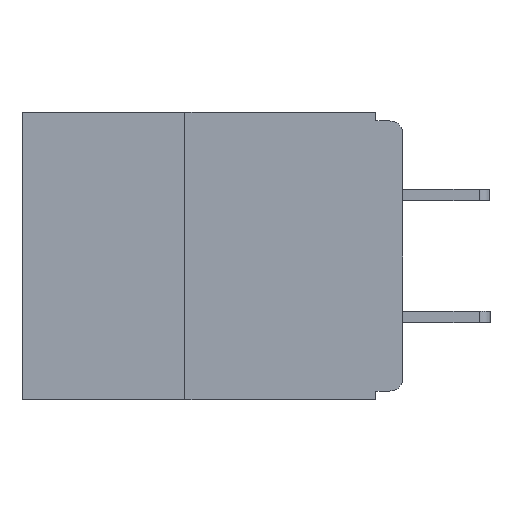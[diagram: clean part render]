
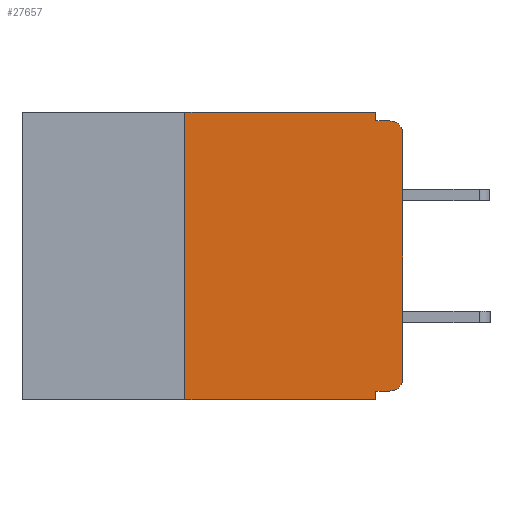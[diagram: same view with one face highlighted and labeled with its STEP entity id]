
A CAD part, left-side view. The second image highlights one B-rep face of the part: STEP entity #27657.
In plain terms, the highlighted planar face has unit normal (-1, 0, 0).
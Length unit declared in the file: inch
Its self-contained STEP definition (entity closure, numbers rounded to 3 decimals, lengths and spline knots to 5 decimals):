
#57 = VECTOR ( 'NONE', #18322, 39.37008 ) ;
#521 = DIRECTION ( 'NONE',  ( 0., 0., -1. ) ) ;
#872 = CARTESIAN_POINT ( 'NONE',  ( 0., 0.015, -0.01 ) ) ;
#1407 = EDGE_CURVE ( 'NONE', #8195, #27030, #6250, .T. ) ;
#2153 = CARTESIAN_POINT ( 'NONE',  ( 0., 0.031, -0.32 ) ) ;
#2713 = ORIENTED_EDGE ( 'NONE', *, *, #29610, .F. ) ;
#2787 = FACE_OUTER_BOUND ( 'NONE', #13685, .T. ) ;
#2951 = VECTOR ( 'NONE', #14646, 39.37008 ) ;
#3457 = DIRECTION ( 'NONE',  ( -1., 0., 0. ) ) ;
#4063 = CIRCLE ( 'NONE', #12499, 0.015 ) ;
#4450 = LINE ( 'NONE', #19213, #10654 ) ;
#4582 = VECTOR ( 'NONE', #12006, 39.37008 ) ;
#4589 = EDGE_CURVE ( 'NONE', #11374, #17692, #28238, .T. ) ;
#4731 = ORIENTED_EDGE ( 'NONE', *, *, #5599, .F. ) ;
#5529 = CARTESIAN_POINT ( 'NONE',  ( 0., 0.437, -0.33 ) ) ;
#5599 = EDGE_CURVE ( 'NONE', #20520, #16499, #4450, .T. ) ;
#5696 = EDGE_CURVE ( 'NONE', #13863, #11374, #8470, .T. ) ;
#5766 = LINE ( 'NONE', #19676, #28654 ) ;
#6149 = ORIENTED_EDGE ( 'NONE', *, *, #15464, .T. ) ;
#6250 = LINE ( 'NONE', #11486, #57 ) ;
#6683 = ORIENTED_EDGE ( 'NONE', *, *, #4589, .F. ) ;
#7742 = VECTOR ( 'NONE', #10347, 39.37008 ) ;
#8195 = VERTEX_POINT ( 'NONE', #14950 ) ;
#8242 = EDGE_CURVE ( 'NONE', #20500, #12302, #5766, .T. ) ;
#8470 = LINE ( 'NONE', #17174, #7742 ) ;
#8773 = ORIENTED_EDGE ( 'NONE', *, *, #5696, .F. ) ;
#9091 = ORIENTED_EDGE ( 'NONE', *, *, #23774, .T. ) ;
#9218 = LINE ( 'NONE', #22849, #20745 ) ;
#9388 = EDGE_CURVE ( 'NONE', #27030, #12302, #15847, .T. ) ;
#10347 = DIRECTION ( 'NONE',  ( 0., 1., 0. ) ) ;
#10654 = VECTOR ( 'NONE', #16890, 39.37008 ) ;
#10794 = CARTESIAN_POINT ( 'NONE',  ( 0., 0., -0.025 ) ) ;
#11280 = DIRECTION ( 'NONE',  ( -1., 0., 0. ) ) ;
#11374 = VERTEX_POINT ( 'NONE', #2153 ) ;
#11486 = CARTESIAN_POINT ( 'NONE',  ( 0., 0., 0. ) ) ;
#11570 = CARTESIAN_POINT ( 'NONE',  ( 0., 0.031, -0.33 ) ) ;
#12006 = DIRECTION ( 'NONE',  ( 0., 0., -1. ) ) ;
#12302 = VERTEX_POINT ( 'NONE', #872 ) ;
#12499 = AXIS2_PLACEMENT_3D ( 'NONE', #17311, #3457, #19650 ) ;
#12978 = AXIS2_PLACEMENT_3D ( 'NONE', #24974, #11280, #27219 ) ;
#13055 = CARTESIAN_POINT ( 'NONE',  ( 0., 0.437, 0. ) ) ;
#13337 = EDGE_CURVE ( 'NONE', #13409, #20500, #29542, .T. ) ;
#13409 = VERTEX_POINT ( 'NONE', #14612 ) ;
#13685 = EDGE_LOOP ( 'NONE', ( #26952, #27055, #28398, #29151, #2713, #4731, #6149, #6683, #8773, #9091 ) ) ;
#13863 = VERTEX_POINT ( 'NONE', #27597 ) ;
#14403 = CARTESIAN_POINT ( 'NONE',  ( 0., 0.031, 0. ) ) ;
#14564 = LINE ( 'NONE', #5529, #2951 ) ;
#14612 = CARTESIAN_POINT ( 'NONE',  ( 0., 0.031, 0. ) ) ;
#14646 = DIRECTION ( 'NONE',  ( 0., -1., 0. ) ) ;
#14950 = CARTESIAN_POINT ( 'NONE',  ( 0., 0., -0.305 ) ) ;
#15394 = DIRECTION ( 'NONE',  ( 0., 0., -1. ) ) ;
#15464 = EDGE_CURVE ( 'NONE', #20520, #17692, #14564, .T. ) ;
#15847 = CIRCLE ( 'NONE', #12978, 0.015 ) ;
#16499 = VERTEX_POINT ( 'NONE', #20814 ) ;
#16890 = DIRECTION ( 'NONE',  ( 0., 0., 1. ) ) ;
#17174 = CARTESIAN_POINT ( 'NONE',  ( 0., 0., -0.32 ) ) ;
#17311 = CARTESIAN_POINT ( 'NONE',  ( 0., 0.015, -0.305 ) ) ;
#17692 = VERTEX_POINT ( 'NONE', #28200 ) ;
#18322 = DIRECTION ( 'NONE',  ( 0., 0., 1. ) ) ;
#18978 = VECTOR ( 'NONE', #521, 39.37008 ) ;
#19213 = CARTESIAN_POINT ( 'NONE',  ( 0., 0.25, -0.33 ) ) ;
#19481 = CARTESIAN_POINT ( 'NONE',  ( 0., 0.031, -0.01 ) ) ;
#19650 = DIRECTION ( 'NONE',  ( 0., 0., -1. ) ) ;
#19676 = CARTESIAN_POINT ( 'NONE',  ( 0., 0., -0.01 ) ) ;
#20500 = VERTEX_POINT ( 'NONE', #19481 ) ;
#20520 = VERTEX_POINT ( 'NONE', #28535 ) ;
#20745 = VECTOR ( 'NONE', #25123, 39.37008 ) ;
#20814 = CARTESIAN_POINT ( 'NONE',  ( 0., 0.25, 0. ) ) ;
#20892 = AXIS2_PLACEMENT_3D ( 'NONE', #13055, #28977, #15394 ) ;
#22849 = CARTESIAN_POINT ( 'NONE',  ( 0., 0.437, 0. ) ) ;
#23774 = EDGE_CURVE ( 'NONE', #13863, #8195, #4063, .T. ) ;
#24974 = CARTESIAN_POINT ( 'NONE',  ( 0., 0.015, -0.025 ) ) ;
#25123 = DIRECTION ( 'NONE',  ( 0., -1., 0. ) ) ;
#26695 = PLANE ( 'NONE',  #20892 ) ;
#26952 = ORIENTED_EDGE ( 'NONE', *, *, #1407, .T. ) ;
#27030 = VERTEX_POINT ( 'NONE', #10794 ) ;
#27055 = ORIENTED_EDGE ( 'NONE', *, *, #9388, .T. ) ;
#27219 = DIRECTION ( 'NONE',  ( 0., 0., -1. ) ) ;
#27597 = CARTESIAN_POINT ( 'NONE',  ( 0., 0.015, -0.32 ) ) ;
#27657 = ADVANCED_FACE ( 'NONE', ( #2787 ), #26695, .F. ) ;
#28200 = CARTESIAN_POINT ( 'NONE',  ( 0., 0.031, -0.33 ) ) ;
#28238 = LINE ( 'NONE', #11570, #4582 ) ;
#28398 = ORIENTED_EDGE ( 'NONE', *, *, #8242, .F. ) ;
#28535 = CARTESIAN_POINT ( 'NONE',  ( 0., 0.25, -0.33 ) ) ;
#28654 = VECTOR ( 'NONE', #28730, 39.37008 ) ;
#28730 = DIRECTION ( 'NONE',  ( 0., -1., 0. ) ) ;
#28977 = DIRECTION ( 'NONE',  ( 1., 0., 0. ) ) ;
#29151 = ORIENTED_EDGE ( 'NONE', *, *, #13337, .F. ) ;
#29542 = LINE ( 'NONE', #14403, #18978 ) ;
#29610 = EDGE_CURVE ( 'NONE', #16499, #13409, #9218, .T. ) ;
